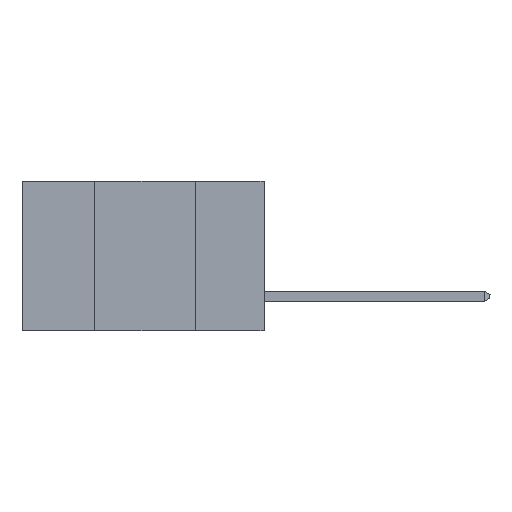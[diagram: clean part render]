
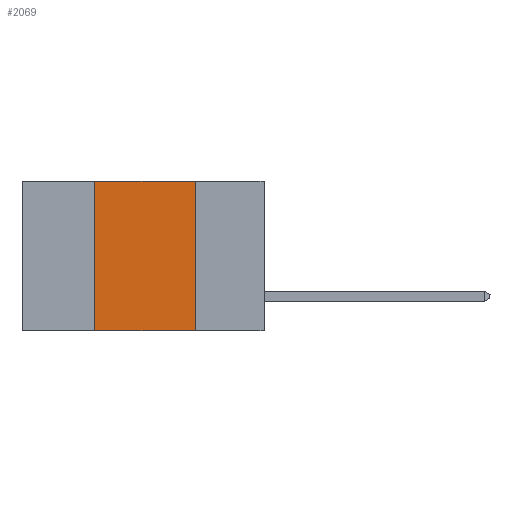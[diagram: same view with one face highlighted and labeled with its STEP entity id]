
A CAD part, left-side view. The second image highlights one B-rep face of the part: STEP entity #2069.
In plain terms, the highlighted planar face has unit normal (-1, 0, 0).
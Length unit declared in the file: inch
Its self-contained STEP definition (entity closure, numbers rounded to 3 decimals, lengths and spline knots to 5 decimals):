
#168 = LINE ( 'NONE', #3689, #5651 ) ;
#193 = ORIENTED_EDGE ( 'NONE', *, *, #14723, .T. ) ;
#555 = CARTESIAN_POINT ( 'NONE',  ( 0., 0.17, -0.37 ) ) ;
#580 = LINE ( 'NONE', #657, #2632 ) ;
#657 = CARTESIAN_POINT ( 'NONE',  ( 0., 0.42, -0.37 ) ) ;
#1061 = EDGE_CURVE ( 'NONE', #8438, #2405, #168, .T. ) ;
#1731 = DIRECTION ( 'NONE',  ( 0., 0., -1. ) ) ;
#1890 = DIRECTION ( 'NONE',  ( 0., -1., 0. ) ) ;
#2066 = EDGE_CURVE ( 'NONE', #4534, #8438, #580, .T. ) ;
#2069 = ADVANCED_FACE ( 'NONE', ( #2868 ), #8666, .F. ) ;
#2325 = ORIENTED_EDGE ( 'NONE', *, *, #1061, .F. ) ;
#2327 = CARTESIAN_POINT ( 'NONE',  ( 0., 0.17, 0. ) ) ;
#2405 = VERTEX_POINT ( 'NONE', #2327 ) ;
#2424 = VECTOR ( 'NONE', #1890, 39.37008 ) ;
#2632 = VECTOR ( 'NONE', #5309, 39.37008 ) ;
#2868 = FACE_OUTER_BOUND ( 'NONE', #6421, .T. ) ;
#3433 = CARTESIAN_POINT ( 'NONE',  ( 0., 0.17, -0.37 ) ) ;
#3502 = ORIENTED_EDGE ( 'NONE', *, *, #9232, .F. ) ;
#3689 = CARTESIAN_POINT ( 'NONE',  ( 0., 0.6, 0. ) ) ;
#3841 = DIRECTION ( 'NONE',  ( 0., -1., 0. ) ) ;
#4534 = VERTEX_POINT ( 'NONE', #13093 ) ;
#5309 = DIRECTION ( 'NONE',  ( 0., 0., 1. ) ) ;
#5508 = CARTESIAN_POINT ( 'NONE',  ( 0., 0.6, 0. ) ) ;
#5651 = VECTOR ( 'NONE', #3841, 39.37008 ) ;
#6192 = DIRECTION ( 'NONE',  ( 0., 0., -1. ) ) ;
#6421 = EDGE_LOOP ( 'NONE', ( #3502, #2325, #14783, #193 ) ) ;
#7601 = DIRECTION ( 'NONE',  ( 1., 0., 0. ) ) ;
#8438 = VERTEX_POINT ( 'NONE', #11287 ) ;
#8638 = VERTEX_POINT ( 'NONE', #3433 ) ;
#8666 = PLANE ( 'NONE',  #12547 ) ;
#9232 = EDGE_CURVE ( 'NONE', #2405, #8638, #10776, .T. ) ;
#9705 = CARTESIAN_POINT ( 'NONE',  ( 0., 0.6, -0.37 ) ) ;
#10776 = LINE ( 'NONE', #555, #12216 ) ;
#11287 = CARTESIAN_POINT ( 'NONE',  ( 0., 0.42, 0. ) ) ;
#12216 = VECTOR ( 'NONE', #6192, 39.37008 ) ;
#12547 = AXIS2_PLACEMENT_3D ( 'NONE', #5508, #7601, #1731 ) ;
#13093 = CARTESIAN_POINT ( 'NONE',  ( 0., 0.42, -0.37 ) ) ;
#14475 = LINE ( 'NONE', #9705, #2424 ) ;
#14723 = EDGE_CURVE ( 'NONE', #4534, #8638, #14475, .T. ) ;
#14783 = ORIENTED_EDGE ( 'NONE', *, *, #2066, .F. ) ;
